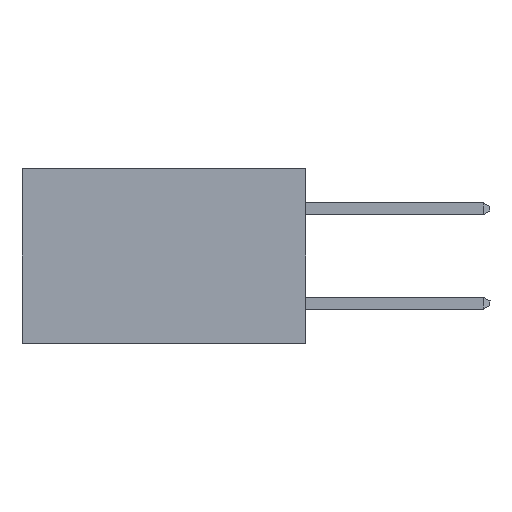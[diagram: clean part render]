
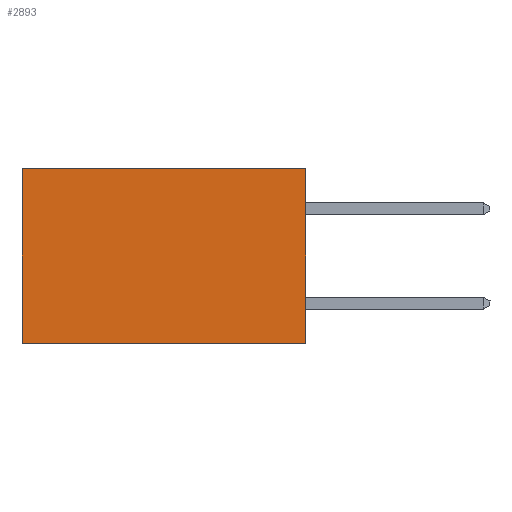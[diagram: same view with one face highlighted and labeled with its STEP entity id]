
A CAD part, left-side view. The second image highlights one B-rep face of the part: STEP entity #2893.
In plain terms, the highlighted planar face has unit normal (-1, 0, 0).
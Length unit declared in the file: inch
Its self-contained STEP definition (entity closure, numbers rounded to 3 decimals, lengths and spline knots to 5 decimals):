
#68 = VERTEX_POINT ( 'NONE', #2023 ) ;
#144 = DIRECTION ( 'NONE',  ( 0., 0., -1. ) ) ;
#251 = EDGE_LOOP ( 'NONE', ( #1945, #2205, #8720, #8211 ) ) ;
#334 = DIRECTION ( 'NONE',  ( 0., 0., -1. ) ) ;
#361 = VERTEX_POINT ( 'NONE', #7511 ) ;
#364 = EDGE_CURVE ( 'NONE', #68, #361, #2272, .T. ) ;
#614 = CARTESIAN_POINT ( 'NONE',  ( 0.298, 0.6, -0.37 ) ) ;
#1012 = EDGE_CURVE ( 'NONE', #361, #7756, #8447, .T. ) ;
#1358 = EDGE_CURVE ( 'NONE', #68, #8723, #4330, .T. ) ;
#1661 = VECTOR ( 'NONE', #5745, 39.37008 ) ;
#1945 = ORIENTED_EDGE ( 'NONE', *, *, #1012, .T. ) ;
#2023 = CARTESIAN_POINT ( 'NONE',  ( 0.298, 0., 0. ) ) ;
#2205 = ORIENTED_EDGE ( 'NONE', *, *, #8662, .F. ) ;
#2272 = LINE ( 'NONE', #8549, #1661 ) ;
#2792 = DIRECTION ( 'NONE',  ( 0., 0., -1. ) ) ;
#2893 = ADVANCED_FACE ( 'NONE', ( #3561 ), #6636, .F. ) ;
#3376 = CARTESIAN_POINT ( 'NONE',  ( 0.298, 0., 0. ) ) ;
#3532 = CARTESIAN_POINT ( 'NONE',  ( 0.298, 0.6, 0. ) ) ;
#3561 = FACE_OUTER_BOUND ( 'NONE', #251, .T. ) ;
#4079 = VECTOR ( 'NONE', #2792, 39.37008 ) ;
#4330 = LINE ( 'NONE', #3376, #8054 ) ;
#5059 = DIRECTION ( 'NONE',  ( 1., 0., 0. ) ) ;
#5745 = DIRECTION ( 'NONE',  ( 0., 1., 0. ) ) ;
#5876 = LINE ( 'NONE', #7483, #9361 ) ;
#5893 = CARTESIAN_POINT ( 'NONE',  ( 0.298, 0., -0.37 ) ) ;
#6636 = PLANE ( 'NONE',  #7962 ) ;
#7483 = CARTESIAN_POINT ( 'NONE',  ( 0.298, 0., -0.37 ) ) ;
#7511 = CARTESIAN_POINT ( 'NONE',  ( 0.298, 0.6, 0. ) ) ;
#7756 = VERTEX_POINT ( 'NONE', #614 ) ;
#7962 = AXIS2_PLACEMENT_3D ( 'NONE', #9049, #5059, #334 ) ;
#8054 = VECTOR ( 'NONE', #144, 39.37008 ) ;
#8211 = ORIENTED_EDGE ( 'NONE', *, *, #364, .T. ) ;
#8248 = DIRECTION ( 'NONE',  ( 0., 1., 0. ) ) ;
#8447 = LINE ( 'NONE', #3532, #4079 ) ;
#8549 = CARTESIAN_POINT ( 'NONE',  ( 0.298, 0., 0. ) ) ;
#8662 = EDGE_CURVE ( 'NONE', #8723, #7756, #5876, .T. ) ;
#8720 = ORIENTED_EDGE ( 'NONE', *, *, #1358, .F. ) ;
#8723 = VERTEX_POINT ( 'NONE', #5893 ) ;
#9049 = CARTESIAN_POINT ( 'NONE',  ( 0.298, 0., 0. ) ) ;
#9361 = VECTOR ( 'NONE', #8248, 39.37008 ) ;
